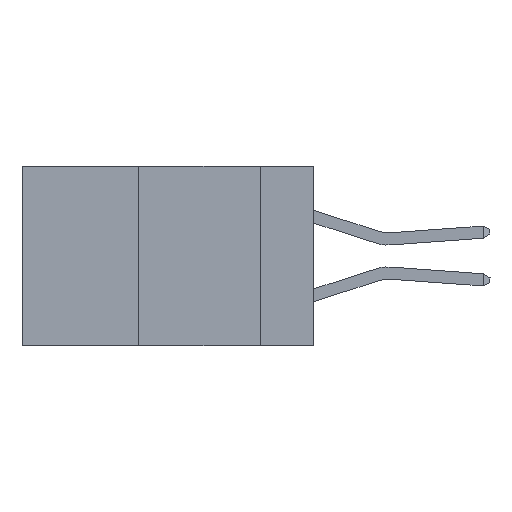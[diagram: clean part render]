
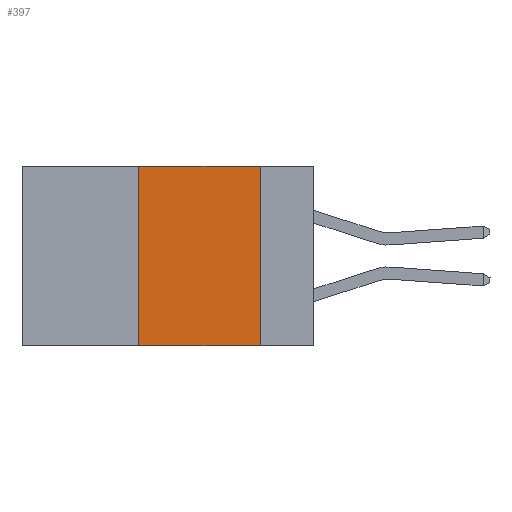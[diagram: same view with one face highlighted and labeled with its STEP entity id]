
A CAD part, left-side view. The second image highlights one B-rep face of the part: STEP entity #397.
In plain terms, the highlighted planar face has unit normal (-1, 0, 0).
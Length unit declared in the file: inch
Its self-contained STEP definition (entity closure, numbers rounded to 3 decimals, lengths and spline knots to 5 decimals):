
#397 = ADVANCED_FACE ( 'NONE', ( #4112 ), #9712, .F. ) ;
#527 = DIRECTION ( 'NONE',  ( 0., 0., -1. ) ) ;
#1057 = CARTESIAN_POINT ( 'NONE',  ( 0., 0.6, 0. ) ) ;
#1077 = ORIENTED_EDGE ( 'NONE', *, *, #1179, .F. ) ;
#1082 = CARTESIAN_POINT ( 'NONE',  ( 0., 0.36, 0. ) ) ;
#1179 = EDGE_CURVE ( 'NONE', #3381, #5733, #10594, .T. ) ;
#1230 = VECTOR ( 'NONE', #527, 39.37008 ) ;
#1260 = ORIENTED_EDGE ( 'NONE', *, *, #7531, .F. ) ;
#1356 = CARTESIAN_POINT ( 'NONE',  ( 0., 0.11, 0. ) ) ;
#1778 = EDGE_CURVE ( 'NONE', #6324, #2861, #5794, .T. ) ;
#2012 = CARTESIAN_POINT ( 'NONE',  ( 0., 0.36, -0.37 ) ) ;
#2066 = LINE ( 'NONE', #1057, #9048 ) ;
#2376 = DIRECTION ( 'NONE',  ( 0., -1., 0. ) ) ;
#2861 = VERTEX_POINT ( 'NONE', #4133 ) ;
#3060 = AXIS2_PLACEMENT_3D ( 'NONE', #5398, #7467, #7013 ) ;
#3381 = VERTEX_POINT ( 'NONE', #7142 ) ;
#4112 = FACE_OUTER_BOUND ( 'NONE', #6340, .T. ) ;
#4133 = CARTESIAN_POINT ( 'NONE',  ( 0., 0.36, 0. ) ) ;
#5129 = ORIENTED_EDGE ( 'NONE', *, *, #1778, .F. ) ;
#5398 = CARTESIAN_POINT ( 'NONE',  ( 0., 0.6, 0. ) ) ;
#5733 = VERTEX_POINT ( 'NONE', #6277 ) ;
#5794 = LINE ( 'NONE', #1082, #10329 ) ;
#6277 = CARTESIAN_POINT ( 'NONE',  ( 0., 0.11, -0.37 ) ) ;
#6324 = VERTEX_POINT ( 'NONE', #2012 ) ;
#6340 = EDGE_LOOP ( 'NONE', ( #1077, #1260, #5129, #6394 ) ) ;
#6394 = ORIENTED_EDGE ( 'NONE', *, *, #6902, .T. ) ;
#6716 = LINE ( 'NONE', #7554, #8611 ) ;
#6902 = EDGE_CURVE ( 'NONE', #6324, #5733, #6716, .T. ) ;
#7013 = DIRECTION ( 'NONE',  ( 0., 0., -1. ) ) ;
#7142 = CARTESIAN_POINT ( 'NONE',  ( 0., 0.11, 0. ) ) ;
#7309 = DIRECTION ( 'NONE',  ( 0., -1., 0. ) ) ;
#7467 = DIRECTION ( 'NONE',  ( 1., 0., 0. ) ) ;
#7531 = EDGE_CURVE ( 'NONE', #2861, #3381, #2066, .T. ) ;
#7554 = CARTESIAN_POINT ( 'NONE',  ( 0., 0.6, -0.37 ) ) ;
#8611 = VECTOR ( 'NONE', #7309, 39.37008 ) ;
#8730 = DIRECTION ( 'NONE',  ( 0., 0., 1. ) ) ;
#9048 = VECTOR ( 'NONE', #2376, 39.37008 ) ;
#9712 = PLANE ( 'NONE',  #3060 ) ;
#10329 = VECTOR ( 'NONE', #8730, 39.37008 ) ;
#10594 = LINE ( 'NONE', #1356, #1230 ) ;
